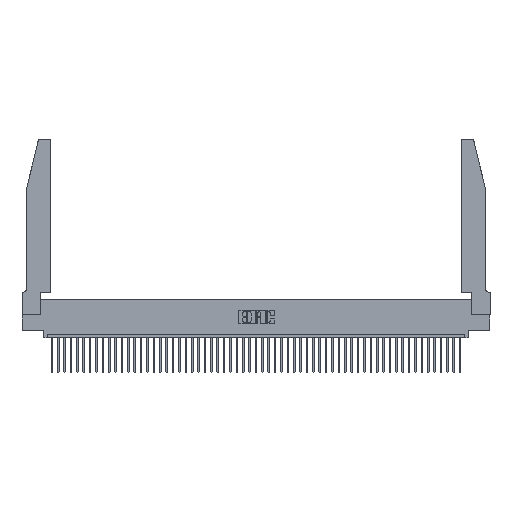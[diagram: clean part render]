
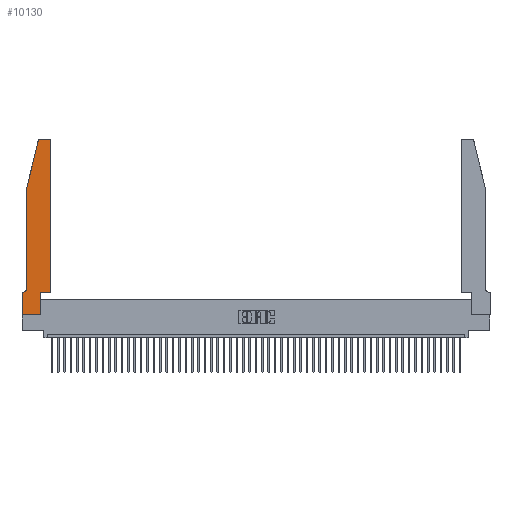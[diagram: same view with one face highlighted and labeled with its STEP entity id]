
A CAD part, top view. The second image highlights one B-rep face of the part: STEP entity #10130.
In plain terms, the highlighted planar face has unit normal (0, 0, 1).
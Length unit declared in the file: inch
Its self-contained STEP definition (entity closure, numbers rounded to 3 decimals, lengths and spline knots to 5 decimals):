
#11 = VERTEX_POINT ( 'NONE', #45432 ) ;
#335 = CARTESIAN_POINT ( 'NONE',  ( 0.4505, 0.35, 0.37 ) ) ;
#1064 = DIRECTION ( 'NONE',  ( -1., 0., 0. ) ) ;
#2393 = CARTESIAN_POINT ( 'NONE',  ( 0.284, 2.72, 0.37 ) ) ;
#2450 = EDGE_CURVE ( 'NONE', #28092, #4660, #20879, .T. ) ;
#3275 = LINE ( 'NONE', #23067, #50386 ) ;
#3749 = CIRCLE ( 'NONE', #49004, 0.07 ) ;
#3762 = CARTESIAN_POINT ( 'NONE',  ( 0.4505, 0.35, 0.37 ) ) ;
#3788 = CARTESIAN_POINT ( 'NONE',  ( 0.2865, 0., 0.37 ) ) ;
#4440 = VERTEX_POINT ( 'NONE', #31142 ) ;
#4475 = VECTOR ( 'NONE', #30265, 39.37008 ) ;
#4660 = VERTEX_POINT ( 'NONE', #18457 ) ;
#4814 = DIRECTION ( 'NONE',  ( 0., 0., 1. ) ) ;
#4829 = EDGE_CURVE ( 'NONE', #23054, #26588, #33129, .T. ) ;
#4904 = LINE ( 'NONE', #18839, #27476 ) ;
#6267 = DIRECTION ( 'NONE',  ( 0., 0., 1. ) ) ;
#7312 = DIRECTION ( 'NONE',  ( 0., -1., 0. ) ) ;
#7744 = DIRECTION ( 'NONE',  ( 0., 1., 0. ) ) ;
#7757 = VERTEX_POINT ( 'NONE', #29647 ) ;
#8253 = AXIS2_PLACEMENT_3D ( 'NONE', #2393, #6267, #31908 ) ;
#9979 = PLANE ( 'NONE',  #41011 ) ;
#10130 = ADVANCED_FACE ( 'NONE', ( #21596 ), #9979, .T. ) ;
#10913 = LINE ( 'NONE', #13976, #26208 ) ;
#11252 = CARTESIAN_POINT ( 'NONE',  ( 0., 0., 0.37 ) ) ;
#12927 = LINE ( 'NONE', #18810, #30696 ) ;
#13212 = CARTESIAN_POINT ( 'NONE',  ( 0.0055, 0.42, 0.37 ) ) ;
#13260 = DIRECTION ( 'NONE',  ( 0., 0., 1. ) ) ;
#13934 = CARTESIAN_POINT ( 'NONE',  ( 0., 0.35, 0.37 ) ) ;
#13976 = CARTESIAN_POINT ( 'NONE',  ( 0.0755, 2., 0.37 ) ) ;
#14653 = VECTOR ( 'NONE', #1064, 39.37008 ) ;
#15127 = VECTOR ( 'NONE', #35074, 39.37008 ) ;
#15725 = EDGE_CURVE ( 'NONE', #26588, #19992, #21252, .T. ) ;
#15952 = EDGE_CURVE ( 'NONE', #26530, #23054, #40963, .T. ) ;
#16055 = CARTESIAN_POINT ( 'NONE',  ( 0.4205, 2.72, 0.37 ) ) ;
#16944 = DIRECTION ( 'NONE',  ( 0., 0., -1. ) ) ;
#17102 = DIRECTION ( 'NONE',  ( -1., 0., 0. ) ) ;
#17705 = VECTOR ( 'NONE', #22796, 39.37008 ) ;
#18457 = CARTESIAN_POINT ( 'NONE',  ( 0.25487, 2.72718, 0.37 ) ) ;
#18643 = DIRECTION ( 'NONE',  ( -1., 0., 0. ) ) ;
#18810 = CARTESIAN_POINT ( 'NONE',  ( 0.2605, 2.75, 0.37 ) ) ;
#18839 = CARTESIAN_POINT ( 'NONE',  ( 0.2865, 0.35, 0.37 ) ) ;
#18897 = DIRECTION ( 'NONE',  ( -0.239, -0.971, 0. ) ) ;
#18947 = CARTESIAN_POINT ( 'NONE',  ( 0.284, 2.75, 0.37 ) ) ;
#19110 = ORIENTED_EDGE ( 'NONE', *, *, #22266, .T. ) ;
#19992 = VERTEX_POINT ( 'NONE', #36641 ) ;
#20339 = CARTESIAN_POINT ( 'NONE',  ( 0.2865, 0.35, 0.37 ) ) ;
#20777 = EDGE_CURVE ( 'NONE', #11, #33893, #35706, .T. ) ;
#20879 = CIRCLE ( 'NONE', #8253, 0.03 ) ;
#21252 = CIRCLE ( 'NONE', #42477, 0.03 ) ;
#21456 = EDGE_CURVE ( 'NONE', #19992, #28092, #12927, .T. ) ;
#21472 = ORIENTED_EDGE ( 'NONE', *, *, #43495, .T. ) ;
#21596 = FACE_OUTER_BOUND ( 'NONE', #38253, .T. ) ;
#22244 = EDGE_CURVE ( 'NONE', #33893, #26530, #4904, .T. ) ;
#22266 = EDGE_CURVE ( 'NONE', #22872, #7757, #47118, .T. ) ;
#22796 = DIRECTION ( 'NONE',  ( 0., -1., 0. ) ) ;
#22872 = VERTEX_POINT ( 'NONE', #49830 ) ;
#23054 = VERTEX_POINT ( 'NONE', #335 ) ;
#23067 = CARTESIAN_POINT ( 'NONE',  ( 0., 0., 0.37 ) ) ;
#23134 = CARTESIAN_POINT ( 'NONE',  ( 0.0755, 2., 0.37 ) ) ;
#23911 = DIRECTION ( 'NONE',  ( 1., 0., 0. ) ) ;
#26208 = VECTOR ( 'NONE', #18897, 39.37008 ) ;
#26530 = VERTEX_POINT ( 'NONE', #20339 ) ;
#26588 = VERTEX_POINT ( 'NONE', #48981 ) ;
#27476 = VECTOR ( 'NONE', #7744, 39.37008 ) ;
#28092 = VERTEX_POINT ( 'NONE', #18947 ) ;
#29325 = DIRECTION ( 'NONE',  ( 1., 0., 0. ) ) ;
#29647 = CARTESIAN_POINT ( 'NONE',  ( 0.0755, 0.42, 0.37 ) ) ;
#29719 = ORIENTED_EDGE ( 'NONE', *, *, #22244, .T. ) ;
#30265 = DIRECTION ( 'NONE',  ( 1., 0., 0. ) ) ;
#30372 = EDGE_CURVE ( 'NONE', #4660, #22872, #10913, .T. ) ;
#30696 = VECTOR ( 'NONE', #18643, 39.37008 ) ;
#31142 = CARTESIAN_POINT ( 'NONE',  ( 0.0055, 0.35, 0.37 ) ) ;
#31908 = DIRECTION ( 'NONE',  ( 1., 0., 0. ) ) ;
#32041 = CARTESIAN_POINT ( 'NONE',  ( 0.0755, 0.35, 0.37 ) ) ;
#33129 = LINE ( 'NONE', #38624, #41764 ) ;
#33893 = VERTEX_POINT ( 'NONE', #3788 ) ;
#34954 = ORIENTED_EDGE ( 'NONE', *, *, #38363, .T. ) ;
#35074 = DIRECTION ( 'NONE',  ( 1., 0., 0. ) ) ;
#35401 = VERTEX_POINT ( 'NONE', #44013 ) ;
#35706 = LINE ( 'NONE', #11252, #4475 ) ;
#36641 = CARTESIAN_POINT ( 'NONE',  ( 0.4205, 2.75, 0.37 ) ) ;
#37280 = ORIENTED_EDGE ( 'NONE', *, *, #2450, .T. ) ;
#38114 = DIRECTION ( 'NONE',  ( 0., 1., 0. ) ) ;
#38253 = EDGE_LOOP ( 'NONE', ( #47244, #37280, #46794, #19110, #34954, #50709, #21472, #42866, #29719, #39352, #47643, #39750 ) ) ;
#38363 = EDGE_CURVE ( 'NONE', #7757, #4440, #3749, .T. ) ;
#38624 = CARTESIAN_POINT ( 'NONE',  ( 0.4505, 0.35, 0.37 ) ) ;
#39352 = ORIENTED_EDGE ( 'NONE', *, *, #15952, .T. ) ;
#39750 = ORIENTED_EDGE ( 'NONE', *, *, #15725, .T. ) ;
#40963 = LINE ( 'NONE', #3762, #15127 ) ;
#41011 = AXIS2_PLACEMENT_3D ( 'NONE', #13934, #13260, #29325 ) ;
#41064 = LINE ( 'NONE', #32041, #14653 ) ;
#41764 = VECTOR ( 'NONE', #38114, 39.37008 ) ;
#42477 = AXIS2_PLACEMENT_3D ( 'NONE', #16055, #4814, #23911 ) ;
#42866 = ORIENTED_EDGE ( 'NONE', *, *, #20777, .T. ) ;
#43495 = EDGE_CURVE ( 'NONE', #35401, #11, #3275, .T. ) ;
#44013 = CARTESIAN_POINT ( 'NONE',  ( 0., 0.35, 0.37 ) ) ;
#45432 = CARTESIAN_POINT ( 'NONE',  ( 0., 0., 0.37 ) ) ;
#46794 = ORIENTED_EDGE ( 'NONE', *, *, #30372, .T. ) ;
#47118 = LINE ( 'NONE', #23134, #17705 ) ;
#47244 = ORIENTED_EDGE ( 'NONE', *, *, #21456, .T. ) ;
#47643 = ORIENTED_EDGE ( 'NONE', *, *, #4829, .T. ) ;
#48347 = EDGE_CURVE ( 'NONE', #4440, #35401, #41064, .T. ) ;
#48981 = CARTESIAN_POINT ( 'NONE',  ( 0.4505, 2.72, 0.37 ) ) ;
#49004 = AXIS2_PLACEMENT_3D ( 'NONE', #13212, #16944, #17102 ) ;
#49830 = CARTESIAN_POINT ( 'NONE',  ( 0.0755, 2., 0.37 ) ) ;
#50386 = VECTOR ( 'NONE', #7312, 39.37008 ) ;
#50709 = ORIENTED_EDGE ( 'NONE', *, *, #48347, .T. ) ;
